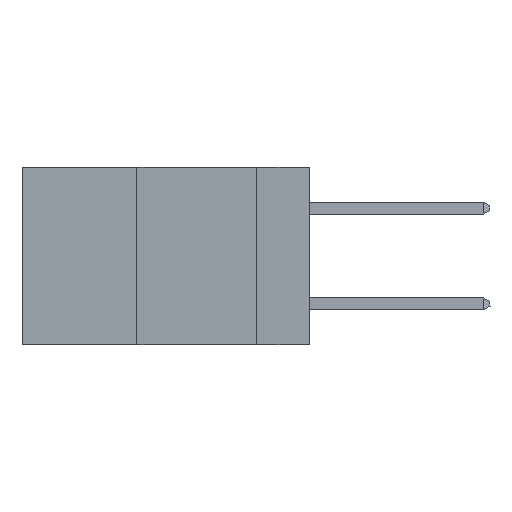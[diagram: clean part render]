
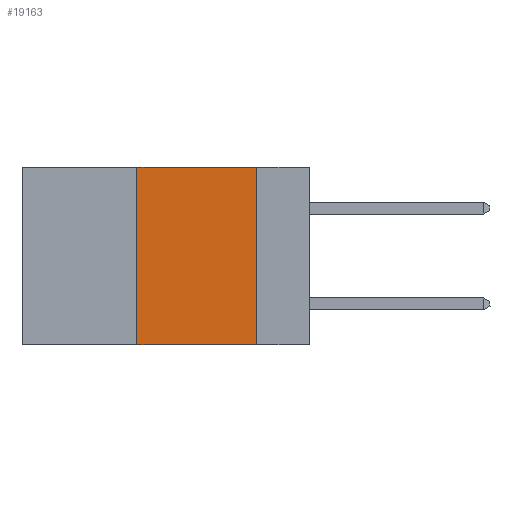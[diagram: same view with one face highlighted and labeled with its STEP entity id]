
A CAD part, left-side view. The second image highlights one B-rep face of the part: STEP entity #19163.
In plain terms, the highlighted planar face has unit normal (-1, 0, 0).
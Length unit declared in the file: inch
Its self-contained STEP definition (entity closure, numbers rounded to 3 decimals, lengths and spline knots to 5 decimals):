
#331 = VERTEX_POINT ( 'NONE', #12313 ) ;
#1678 = VERTEX_POINT ( 'NONE', #23405 ) ;
#2922 = EDGE_CURVE ( 'NONE', #9620, #14243, #17124, .T. ) ;
#4197 = DIRECTION ( 'NONE',  ( 0., 0., 1. ) ) ;
#6130 = DIRECTION ( 'NONE',  ( 1., 0., 0. ) ) ;
#8360 = VECTOR ( 'NONE', #11603, 39.37008 ) ;
#9620 = VERTEX_POINT ( 'NONE', #12105 ) ;
#9833 = EDGE_CURVE ( 'NONE', #331, #1678, #23281, .T. ) ;
#10110 = CARTESIAN_POINT ( 'NONE',  ( 0., 0.6, -0.37 ) ) ;
#11425 = CARTESIAN_POINT ( 'NONE',  ( 0., 0.36, 0. ) ) ;
#11603 = DIRECTION ( 'NONE',  ( 0., -1., 0. ) ) ;
#12105 = CARTESIAN_POINT ( 'NONE',  ( 0., 0.36, -0.37 ) ) ;
#12313 = CARTESIAN_POINT ( 'NONE',  ( 0., 0.11, 0. ) ) ;
#12690 = LINE ( 'NONE', #22569, #8360 ) ;
#12958 = AXIS2_PLACEMENT_3D ( 'NONE', #13432, #6130, #18903 ) ;
#13226 = VECTOR ( 'NONE', #13977, 39.37008 ) ;
#13432 = CARTESIAN_POINT ( 'NONE',  ( 0., 0.6, 0. ) ) ;
#13977 = DIRECTION ( 'NONE',  ( 0., -1., 0. ) ) ;
#14243 = VERTEX_POINT ( 'NONE', #22645 ) ;
#16519 = DIRECTION ( 'NONE',  ( 0., 0., -1. ) ) ;
#17092 = PLANE ( 'NONE',  #12958 ) ;
#17124 = LINE ( 'NONE', #11425, #21382 ) ;
#17450 = VECTOR ( 'NONE', #16519, 39.37008 ) ;
#18072 = LINE ( 'NONE', #10110, #13226 ) ;
#18698 = ORIENTED_EDGE ( 'NONE', *, *, #19169, .F. ) ;
#18784 = ORIENTED_EDGE ( 'NONE', *, *, #2922, .F. ) ;
#18903 = DIRECTION ( 'NONE',  ( 0., 0., -1. ) ) ;
#19163 = ADVANCED_FACE ( 'NONE', ( #23507 ), #17092, .F. ) ;
#19169 = EDGE_CURVE ( 'NONE', #14243, #331, #12690, .T. ) ;
#19988 = EDGE_CURVE ( 'NONE', #9620, #1678, #18072, .T. ) ;
#21382 = VECTOR ( 'NONE', #4197, 39.37008 ) ;
#21452 = ORIENTED_EDGE ( 'NONE', *, *, #19988, .T. ) ;
#21837 = CARTESIAN_POINT ( 'NONE',  ( 0., 0.11, 0. ) ) ;
#22267 = EDGE_LOOP ( 'NONE', ( #22607, #18698, #18784, #21452 ) ) ;
#22569 = CARTESIAN_POINT ( 'NONE',  ( 0., 0.6, 0. ) ) ;
#22607 = ORIENTED_EDGE ( 'NONE', *, *, #9833, .F. ) ;
#22645 = CARTESIAN_POINT ( 'NONE',  ( 0., 0.36, 0. ) ) ;
#23281 = LINE ( 'NONE', #21837, #17450 ) ;
#23405 = CARTESIAN_POINT ( 'NONE',  ( 0., 0.11, -0.37 ) ) ;
#23507 = FACE_OUTER_BOUND ( 'NONE', #22267, .T. ) ;
